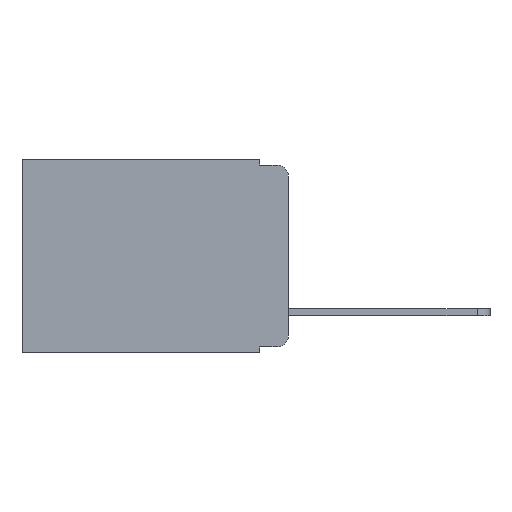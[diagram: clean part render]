
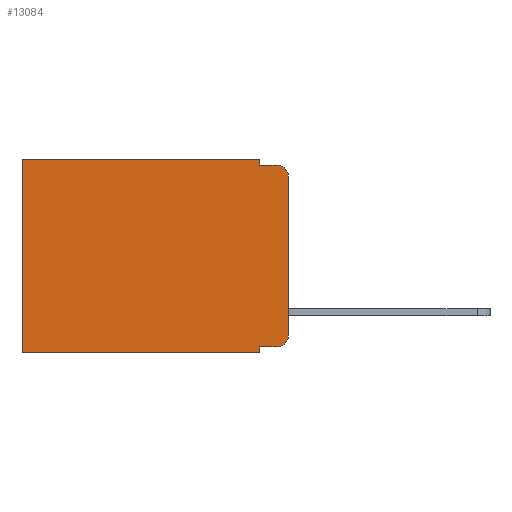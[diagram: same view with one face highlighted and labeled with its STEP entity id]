
A CAD part, left-side view. The second image highlights one B-rep face of the part: STEP entity #13084.
In plain terms, the highlighted planar face has unit normal (-1, 0, 0).
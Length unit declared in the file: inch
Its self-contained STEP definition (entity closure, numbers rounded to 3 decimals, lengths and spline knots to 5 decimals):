
#76 = LINE ( 'NONE', #13794, #3656 ) ;
#477 = CARTESIAN_POINT ( 'NONE',  ( 0.298, 0.473, -0.343 ) ) ;
#554 = VERTEX_POINT ( 'NONE', #14170 ) ;
#733 = DIRECTION ( 'NONE',  ( 0., 0., -1. ) ) ;
#857 = VERTEX_POINT ( 'NONE', #13876 ) ;
#1368 = ORIENTED_EDGE ( 'NONE', *, *, #5407, .T. ) ;
#1377 = DIRECTION ( 'NONE',  ( 0., 0., -1. ) ) ;
#1412 = VERTEX_POINT ( 'NONE', #9621 ) ;
#1538 = VERTEX_POINT ( 'NONE', #11573 ) ;
#1857 = LINE ( 'NONE', #12508, #15787 ) ;
#1928 = LINE ( 'NONE', #5861, #2873 ) ;
#2200 = PLANE ( 'NONE',  #18338 ) ;
#2612 = CARTESIAN_POINT ( 'NONE',  ( 0.298, 0.02, -0.313 ) ) ;
#2873 = VECTOR ( 'NONE', #15833, 39.37008 ) ;
#3005 = CIRCLE ( 'NONE', #14180, 0.02 ) ;
#3473 = EDGE_CURVE ( 'NONE', #554, #3485, #12170, .T. ) ;
#3485 = VERTEX_POINT ( 'NONE', #17753 ) ;
#3626 = CARTESIAN_POINT ( 'NONE',  ( 0.298, 0., 0. ) ) ;
#3656 = VECTOR ( 'NONE', #17891, 39.37008 ) ;
#3691 = DIRECTION ( 'NONE',  ( 0., 0., -1. ) ) ;
#3901 = VECTOR ( 'NONE', #6476, 39.37008 ) ;
#3938 = ORIENTED_EDGE ( 'NONE', *, *, #12187, .F. ) ;
#4066 = DIRECTION ( 'NONE',  ( 0., 0., -1. ) ) ;
#4163 = ORIENTED_EDGE ( 'NONE', *, *, #16265, .T. ) ;
#4209 = CARTESIAN_POINT ( 'NONE',  ( 0.298, 0.051, -0.01 ) ) ;
#4810 = EDGE_CURVE ( 'NONE', #1538, #6353, #18398, .T. ) ;
#5387 = CARTESIAN_POINT ( 'NONE',  ( 0.298, 0.051, -0.01 ) ) ;
#5407 = EDGE_CURVE ( 'NONE', #6353, #10479, #1857, .T. ) ;
#5419 = EDGE_LOOP ( 'NONE', ( #3938, #12081, #8291, #12535, #16657, #1368, #9614, #17069, #4163, #17507 ) ) ;
#5692 = DIRECTION ( 'NONE',  ( 0., -1., 0. ) ) ;
#5861 = CARTESIAN_POINT ( 'NONE',  ( 0.298, 0., 0. ) ) ;
#6353 = VERTEX_POINT ( 'NONE', #13943 ) ;
#6378 = EDGE_CURVE ( 'NONE', #1538, #12128, #14900, .T. ) ;
#6476 = DIRECTION ( 'NONE',  ( 0., 0., -1. ) ) ;
#6642 = EDGE_CURVE ( 'NONE', #3485, #10479, #15105, .T. ) ;
#6698 = VECTOR ( 'NONE', #15304, 39.37008 ) ;
#7307 = CIRCLE ( 'NONE', #9377, 0.02 ) ;
#7601 = DIRECTION ( 'NONE',  ( 0., 1., 0. ) ) ;
#7732 = VECTOR ( 'NONE', #5692, 39.37008 ) ;
#7927 = CARTESIAN_POINT ( 'NONE',  ( 0.298, 0.051, 0. ) ) ;
#7943 = VERTEX_POINT ( 'NONE', #14418 ) ;
#7946 = CARTESIAN_POINT ( 'NONE',  ( 0.298, 0., 0. ) ) ;
#8291 = ORIENTED_EDGE ( 'NONE', *, *, #8353, .F. ) ;
#8353 = EDGE_CURVE ( 'NONE', #12128, #7943, #11540, .T. ) ;
#9200 = FACE_OUTER_BOUND ( 'NONE', #5419, .T. ) ;
#9300 = EDGE_CURVE ( 'NONE', #857, #7943, #7307, .T. ) ;
#9329 = CARTESIAN_POINT ( 'NONE',  ( 0.298, 0.051, 0. ) ) ;
#9377 = AXIS2_PLACEMENT_3D ( 'NONE', #17931, #9527, #733 ) ;
#9527 = DIRECTION ( 'NONE',  ( -1., 0., 0. ) ) ;
#9614 = ORIENTED_EDGE ( 'NONE', *, *, #6642, .F. ) ;
#9621 = CARTESIAN_POINT ( 'NONE',  ( 0.298, 0.02, -0.333 ) ) ;
#10479 = VERTEX_POINT ( 'NONE', #477 ) ;
#11540 = LINE ( 'NONE', #5387, #7732 ) ;
#11573 = CARTESIAN_POINT ( 'NONE',  ( 0.298, 0.051, 0. ) ) ;
#12081 = ORIENTED_EDGE ( 'NONE', *, *, #9300, .T. ) ;
#12128 = VERTEX_POINT ( 'NONE', #4209 ) ;
#12170 = LINE ( 'NONE', #7927, #16313 ) ;
#12187 = EDGE_CURVE ( 'NONE', #857, #17996, #1928, .T. ) ;
#12340 = DIRECTION ( 'NONE',  ( 1., 0., 0. ) ) ;
#12508 = CARTESIAN_POINT ( 'NONE',  ( 0.298, 0.473, 0. ) ) ;
#12535 = ORIENTED_EDGE ( 'NONE', *, *, #6378, .F. ) ;
#12740 = DIRECTION ( 'NONE',  ( -1., 0., 0. ) ) ;
#13084 = ADVANCED_FACE ( 'NONE', ( #9200 ), #2200, .F. ) ;
#13794 = CARTESIAN_POINT ( 'NONE',  ( 0.298, 0.051, -0.333 ) ) ;
#13876 = CARTESIAN_POINT ( 'NONE',  ( 0.298, 0., -0.03 ) ) ;
#13943 = CARTESIAN_POINT ( 'NONE',  ( 0.298, 0.473, 0. ) ) ;
#14170 = CARTESIAN_POINT ( 'NONE',  ( 0.298, 0.051, -0.333 ) ) ;
#14180 = AXIS2_PLACEMENT_3D ( 'NONE', #2612, #12740, #4066 ) ;
#14392 = EDGE_CURVE ( 'NONE', #1412, #17996, #3005, .T. ) ;
#14418 = CARTESIAN_POINT ( 'NONE',  ( 0.298, 0.02, -0.01 ) ) ;
#14509 = CARTESIAN_POINT ( 'NONE',  ( 0.298, 0., -0.313 ) ) ;
#14900 = LINE ( 'NONE', #9329, #3901 ) ;
#15105 = LINE ( 'NONE', #17439, #17899 ) ;
#15304 = DIRECTION ( 'NONE',  ( 0., 1., 0. ) ) ;
#15787 = VECTOR ( 'NONE', #1377, 39.37008 ) ;
#15833 = DIRECTION ( 'NONE',  ( 0., 0., -1. ) ) ;
#16265 = EDGE_CURVE ( 'NONE', #554, #1412, #76, .T. ) ;
#16313 = VECTOR ( 'NONE', #16383, 39.37008 ) ;
#16383 = DIRECTION ( 'NONE',  ( 0., 0., -1. ) ) ;
#16657 = ORIENTED_EDGE ( 'NONE', *, *, #4810, .T. ) ;
#17069 = ORIENTED_EDGE ( 'NONE', *, *, #3473, .F. ) ;
#17439 = CARTESIAN_POINT ( 'NONE',  ( 0.298, 0., -0.343 ) ) ;
#17507 = ORIENTED_EDGE ( 'NONE', *, *, #14392, .T. ) ;
#17753 = CARTESIAN_POINT ( 'NONE',  ( 0.298, 0.051, -0.343 ) ) ;
#17891 = DIRECTION ( 'NONE',  ( 0., -1., 0. ) ) ;
#17899 = VECTOR ( 'NONE', #7601, 39.37008 ) ;
#17931 = CARTESIAN_POINT ( 'NONE',  ( 0.298, 0.02, -0.03 ) ) ;
#17996 = VERTEX_POINT ( 'NONE', #14509 ) ;
#18338 = AXIS2_PLACEMENT_3D ( 'NONE', #3626, #12340, #3691 ) ;
#18398 = LINE ( 'NONE', #7946, #6698 ) ;
